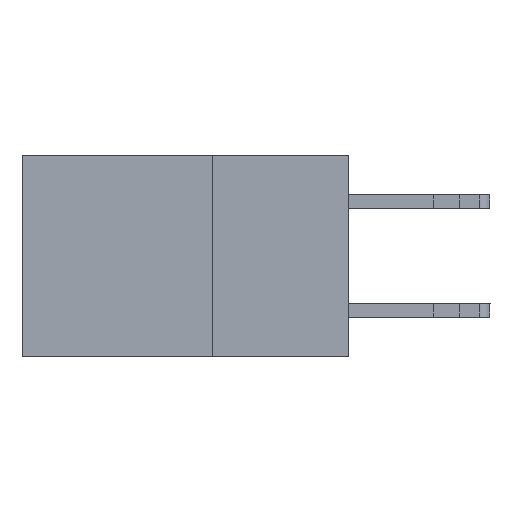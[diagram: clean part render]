
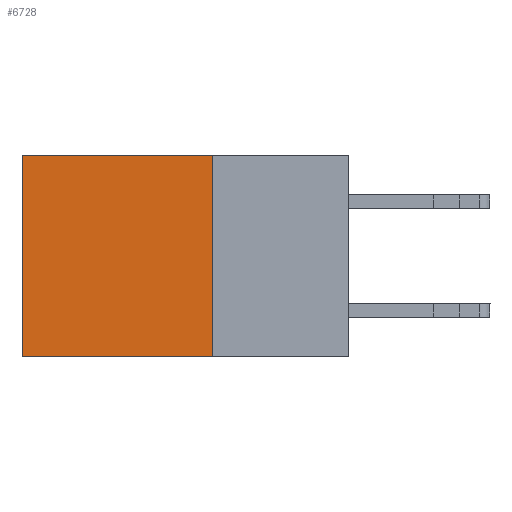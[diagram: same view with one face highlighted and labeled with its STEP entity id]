
A CAD part, left-side view. The second image highlights one B-rep face of the part: STEP entity #6728.
In plain terms, the highlighted planar face has unit normal (-1, 0, 0).
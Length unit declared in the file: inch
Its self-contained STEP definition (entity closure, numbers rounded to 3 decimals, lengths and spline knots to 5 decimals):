
#201 = CARTESIAN_POINT ( 'NONE',  ( 0.298, 0.25, -0.37 ) ) ;
#265 = VECTOR ( 'NONE', #15722, 39.37008 ) ;
#1734 = DIRECTION ( 'NONE',  ( 0., 1., 0. ) ) ;
#2324 = CARTESIAN_POINT ( 'NONE',  ( 0.298, 0.25, 0. ) ) ;
#3276 = LINE ( 'NONE', #11513, #16945 ) ;
#3630 = FACE_OUTER_BOUND ( 'NONE', #12743, .T. ) ;
#4366 = VERTEX_POINT ( 'NONE', #2324 ) ;
#4406 = DIRECTION ( 'NONE',  ( 0., 0., -1. ) ) ;
#4899 = LINE ( 'NONE', #7860, #265 ) ;
#6728 = ADVANCED_FACE ( 'NONE', ( #3630 ), #16714, .F. ) ;
#7359 = CARTESIAN_POINT ( 'NONE',  ( 0.298, 0.25, 0. ) ) ;
#7860 = CARTESIAN_POINT ( 'NONE',  ( 0.298, 0.6, 0. ) ) ;
#9060 = EDGE_CURVE ( 'NONE', #4366, #17322, #3276, .T. ) ;
#9125 = DIRECTION ( 'NONE',  ( 0., 0., -1. ) ) ;
#9194 = ORIENTED_EDGE ( 'NONE', *, *, #16309, .F. ) ;
#9376 = LINE ( 'NONE', #201, #13058 ) ;
#9819 = DIRECTION ( 'NONE',  ( 0., 1., 0. ) ) ;
#11156 = EDGE_CURVE ( 'NONE', #4366, #17080, #19134, .T. ) ;
#11513 = CARTESIAN_POINT ( 'NONE',  ( 0.298, 0.25, 0. ) ) ;
#12349 = EDGE_CURVE ( 'NONE', #17322, #15405, #4899, .T. ) ;
#12372 = CARTESIAN_POINT ( 'NONE',  ( 0.298, 0.6, 0. ) ) ;
#12509 = ORIENTED_EDGE ( 'NONE', *, *, #9060, .T. ) ;
#12743 = EDGE_LOOP ( 'NONE', ( #15068, #9194, #17421, #12509 ) ) ;
#13058 = VECTOR ( 'NONE', #1734, 39.37008 ) ;
#14267 = VECTOR ( 'NONE', #9125, 39.37008 ) ;
#15068 = ORIENTED_EDGE ( 'NONE', *, *, #12349, .T. ) ;
#15405 = VERTEX_POINT ( 'NONE', #19148 ) ;
#15702 = AXIS2_PLACEMENT_3D ( 'NONE', #7359, #20012, #4406 ) ;
#15722 = DIRECTION ( 'NONE',  ( 0., 0., -1. ) ) ;
#16309 = EDGE_CURVE ( 'NONE', #17080, #15405, #9376, .T. ) ;
#16714 = PLANE ( 'NONE',  #15702 ) ;
#16945 = VECTOR ( 'NONE', #9819, 39.37008 ) ;
#17080 = VERTEX_POINT ( 'NONE', #18470 ) ;
#17322 = VERTEX_POINT ( 'NONE', #12372 ) ;
#17421 = ORIENTED_EDGE ( 'NONE', *, *, #11156, .F. ) ;
#18455 = CARTESIAN_POINT ( 'NONE',  ( 0.298, 0.25, 0. ) ) ;
#18470 = CARTESIAN_POINT ( 'NONE',  ( 0.298, 0.25, -0.37 ) ) ;
#19134 = LINE ( 'NONE', #18455, #14267 ) ;
#19148 = CARTESIAN_POINT ( 'NONE',  ( 0.298, 0.6, -0.37 ) ) ;
#20012 = DIRECTION ( 'NONE',  ( 1., 0., 0. ) ) ;
